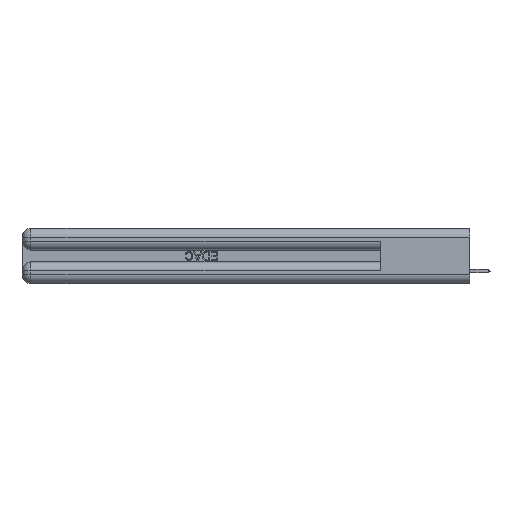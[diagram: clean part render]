
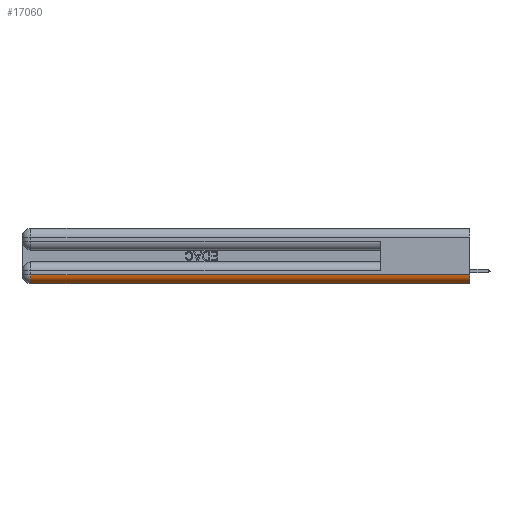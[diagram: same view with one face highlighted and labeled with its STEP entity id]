
A CAD part, left-side view. The second image highlights one B-rep face of the part: STEP entity #17060.
In plain terms, the highlighted cylindrical face has radius 1.524 mm (diameter 3.048 mm), a partial arc.
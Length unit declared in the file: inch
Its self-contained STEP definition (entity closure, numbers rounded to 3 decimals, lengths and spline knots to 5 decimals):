
#3 = EDGE_LOOP ( 'NONE', ( #12229, #30011, #25244, #16549 ) ) ;
#669 = VERTEX_POINT ( 'NONE', #21279 ) ;
#1441 = EDGE_CURVE ( 'NONE', #669, #7670, #10341, .T. ) ;
#1452 = DIRECTION ( 'NONE',  ( 0., 0., 1. ) ) ;
#6624 = AXIS2_PLACEMENT_3D ( 'NONE', #21604, #9499, #31693 ) ;
#6643 = CARTESIAN_POINT ( 'NONE',  ( 0.06, 2.94, 0.06 ) ) ;
#7670 = VERTEX_POINT ( 'NONE', #12185 ) ;
#7951 = AXIS2_PLACEMENT_3D ( 'NONE', #6643, #35180, #32164 ) ;
#9499 = DIRECTION ( 'NONE',  ( 0., 1., 0. ) ) ;
#10341 = CIRCLE ( 'NONE', #7951, 0.06 ) ;
#11447 = CARTESIAN_POINT ( 'NONE',  ( 0.06, 0., 0.06 ) ) ;
#11903 = CARTESIAN_POINT ( 'NONE',  ( 0., 0., 0.06 ) ) ;
#12185 = CARTESIAN_POINT ( 'NONE',  ( 0., 2.94, 0.06 ) ) ;
#12229 = ORIENTED_EDGE ( 'NONE', *, *, #39098, .F. ) ;
#12262 = AXIS2_PLACEMENT_3D ( 'NONE', #11447, #33403, #1452 ) ;
#12312 = VECTOR ( 'NONE', #34241, 39.37008 ) ;
#13511 = CARTESIAN_POINT ( 'NONE',  ( 0.06, 0., 0. ) ) ;
#14254 = LINE ( 'NONE', #11903, #12312 ) ;
#16030 = VERTEX_POINT ( 'NONE', #29597 ) ;
#16549 = ORIENTED_EDGE ( 'NONE', *, *, #24565, .F. ) ;
#17060 = ADVANCED_FACE ( 'NONE', ( #18546 ), #18032, .T. ) ;
#18032 = CYLINDRICAL_SURFACE ( 'NONE', #6624, 0.06 ) ;
#18546 = FACE_OUTER_BOUND ( 'NONE', #3, .T. ) ;
#18732 = CARTESIAN_POINT ( 'NONE',  ( 0.06, 3., 0. ) ) ;
#19391 = DIRECTION ( 'NONE',  ( 0., 1., 0. ) ) ;
#21279 = CARTESIAN_POINT ( 'NONE',  ( 0.06, 2.94, 0. ) ) ;
#21604 = CARTESIAN_POINT ( 'NONE',  ( 0.06, 0., 0.06 ) ) ;
#23226 = VECTOR ( 'NONE', #19391, 39.37008 ) ;
#24565 = EDGE_CURVE ( 'NONE', #35941, #669, #31674, .T. ) ;
#25244 = ORIENTED_EDGE ( 'NONE', *, *, #1441, .F. ) ;
#29597 = CARTESIAN_POINT ( 'NONE',  ( 0., 0., 0.06 ) ) ;
#30011 = ORIENTED_EDGE ( 'NONE', *, *, #31122, .F. ) ;
#31122 = EDGE_CURVE ( 'NONE', #7670, #16030, #14254, .T. ) ;
#31674 = LINE ( 'NONE', #18732, #23226 ) ;
#31693 = DIRECTION ( 'NONE',  ( 0., 0., 1. ) ) ;
#32164 = DIRECTION ( 'NONE',  ( 0., 0., 1. ) ) ;
#33403 = DIRECTION ( 'NONE',  ( 0., -1., 0. ) ) ;
#34241 = DIRECTION ( 'NONE',  ( 0., -1., 0. ) ) ;
#35180 = DIRECTION ( 'NONE',  ( 0., 1., 0. ) ) ;
#35941 = VERTEX_POINT ( 'NONE', #13511 ) ;
#37070 = CIRCLE ( 'NONE', #12262, 0.06 ) ;
#39098 = EDGE_CURVE ( 'NONE', #16030, #35941, #37070, .T. ) ;
